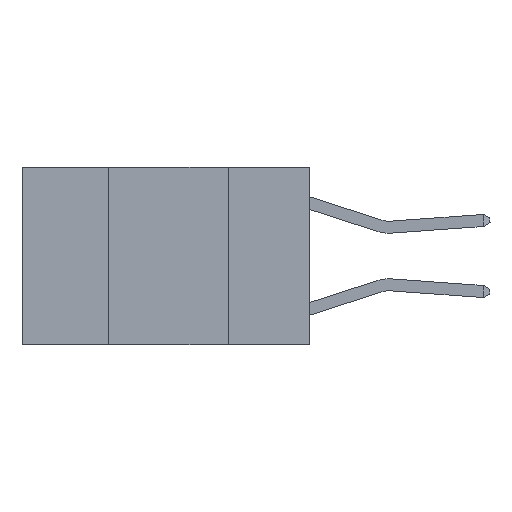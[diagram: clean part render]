
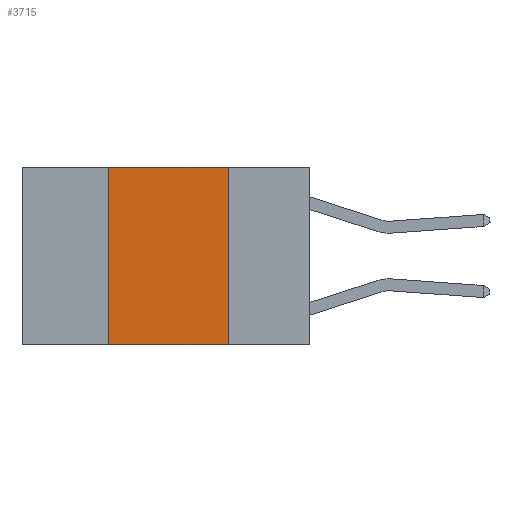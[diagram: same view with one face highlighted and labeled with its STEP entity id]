
A CAD part, left-side view. The second image highlights one B-rep face of the part: STEP entity #3715.
In plain terms, the highlighted planar face has unit normal (-1, 0, 0).
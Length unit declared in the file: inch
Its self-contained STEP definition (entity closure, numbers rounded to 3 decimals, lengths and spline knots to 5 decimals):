
#51 = CARTESIAN_POINT ( 'NONE',  ( 0., 0.6, -0.37 ) ) ;
#215 = AXIS2_PLACEMENT_3D ( 'NONE', #11019, #7801, #2738 ) ;
#940 = CARTESIAN_POINT ( 'NONE',  ( 0., 0.17, -0.37 ) ) ;
#1057 = CARTESIAN_POINT ( 'NONE',  ( 0., 0.42, -0.37 ) ) ;
#1178 = FACE_OUTER_BOUND ( 'NONE', #2981, .T. ) ;
#1835 = PLANE ( 'NONE',  #215 ) ;
#1965 = DIRECTION ( 'NONE',  ( 0., 0., 1. ) ) ;
#1969 = CARTESIAN_POINT ( 'NONE',  ( 0., 0.6, 0. ) ) ;
#2190 = CARTESIAN_POINT ( 'NONE',  ( 0., 0.42, 0. ) ) ;
#2228 = VERTEX_POINT ( 'NONE', #940 ) ;
#2515 = VECTOR ( 'NONE', #8766, 39.37008 ) ;
#2678 = EDGE_CURVE ( 'NONE', #5711, #7683, #6647, .T. ) ;
#2738 = DIRECTION ( 'NONE',  ( 0., 0., -1. ) ) ;
#2805 = VECTOR ( 'NONE', #1965, 39.37008 ) ;
#2981 = EDGE_LOOP ( 'NONE', ( #9319, #6081, #6333, #4084 ) ) ;
#3672 = CARTESIAN_POINT ( 'NONE',  ( 0., 0.17, 0. ) ) ;
#3715 = ADVANCED_FACE ( 'NONE', ( #1178 ), #1835, .F. ) ;
#3885 = VERTEX_POINT ( 'NONE', #1057 ) ;
#4084 = ORIENTED_EDGE ( 'NONE', *, *, #11041, .T. ) ;
#4801 = LINE ( 'NONE', #51, #2515 ) ;
#5711 = VERTEX_POINT ( 'NONE', #2190 ) ;
#6081 = ORIENTED_EDGE ( 'NONE', *, *, #2678, .F. ) ;
#6333 = ORIENTED_EDGE ( 'NONE', *, *, #11026, .F. ) ;
#6647 = LINE ( 'NONE', #1969, #8617 ) ;
#7066 = CARTESIAN_POINT ( 'NONE',  ( 0., 0.42, 0. ) ) ;
#7683 = VERTEX_POINT ( 'NONE', #9633 ) ;
#7801 = DIRECTION ( 'NONE',  ( 1., 0., 0. ) ) ;
#7828 = VECTOR ( 'NONE', #9514, 39.37008 ) ;
#8617 = VECTOR ( 'NONE', #9688, 39.37008 ) ;
#8766 = DIRECTION ( 'NONE',  ( 0., -1., 0. ) ) ;
#9319 = ORIENTED_EDGE ( 'NONE', *, *, #10990, .F. ) ;
#9499 = LINE ( 'NONE', #7066, #2805 ) ;
#9514 = DIRECTION ( 'NONE',  ( 0., 0., -1. ) ) ;
#9633 = CARTESIAN_POINT ( 'NONE',  ( 0., 0.17, 0. ) ) ;
#9688 = DIRECTION ( 'NONE',  ( 0., -1., 0. ) ) ;
#9745 = LINE ( 'NONE', #3672, #7828 ) ;
#10990 = EDGE_CURVE ( 'NONE', #7683, #2228, #9745, .T. ) ;
#11019 = CARTESIAN_POINT ( 'NONE',  ( 0., 0.6, 0. ) ) ;
#11026 = EDGE_CURVE ( 'NONE', #3885, #5711, #9499, .T. ) ;
#11041 = EDGE_CURVE ( 'NONE', #3885, #2228, #4801, .T. ) ;
